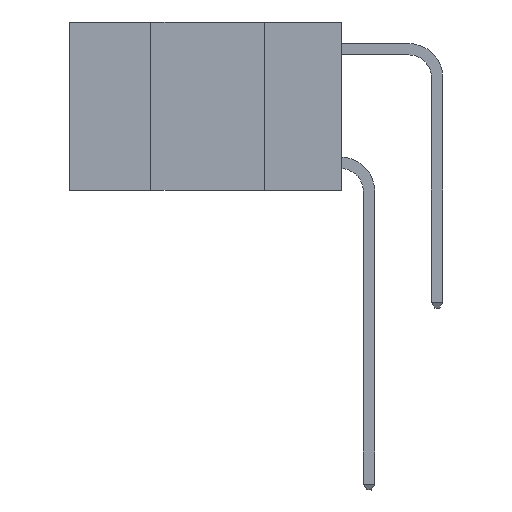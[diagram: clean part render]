
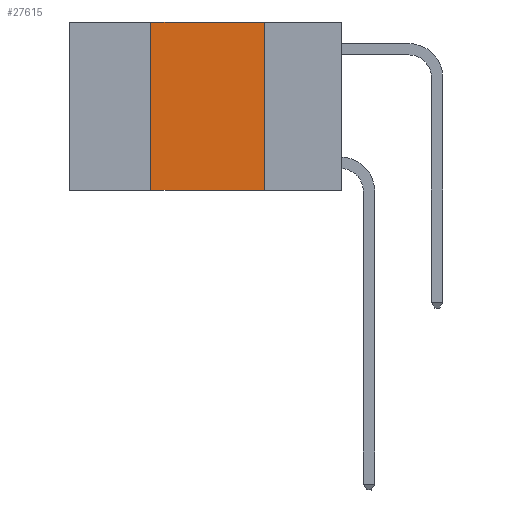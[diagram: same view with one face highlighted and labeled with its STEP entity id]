
A CAD part, left-side view. The second image highlights one B-rep face of the part: STEP entity #27615.
In plain terms, the highlighted planar face has unit normal (-1, 0, 0).
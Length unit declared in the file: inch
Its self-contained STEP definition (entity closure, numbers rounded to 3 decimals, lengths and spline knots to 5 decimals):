
#727 = CARTESIAN_POINT ( 'NONE',  ( 0., 0.6, 0. ) ) ;
#2746 = CARTESIAN_POINT ( 'NONE',  ( 0., 0.17, -0.37 ) ) ;
#2922 = CARTESIAN_POINT ( 'NONE',  ( 0., 0.17, 0. ) ) ;
#3463 = DIRECTION ( 'NONE',  ( 0., 0., -1. ) ) ;
#4274 = DIRECTION ( 'NONE',  ( 0., 0., -1. ) ) ;
#4362 = EDGE_CURVE ( 'NONE', #26511, #19978, #22070, .T. ) ;
#5049 = CARTESIAN_POINT ( 'NONE',  ( 0., 0.6, -0.37 ) ) ;
#6736 = LINE ( 'NONE', #5049, #15609 ) ;
#6961 = CARTESIAN_POINT ( 'NONE',  ( 0., 0.42, -0.37 ) ) ;
#8359 = VECTOR ( 'NONE', #17853, 39.37008 ) ;
#8516 = EDGE_CURVE ( 'NONE', #19978, #18328, #14137, .T. ) ;
#8931 = ORIENTED_EDGE ( 'NONE', *, *, #4362, .F. ) ;
#9910 = EDGE_LOOP ( 'NONE', ( #20988, #8931, #26822, #24869 ) ) ;
#10308 = CARTESIAN_POINT ( 'NONE',  ( 0., 0.6, 0. ) ) ;
#10584 = PLANE ( 'NONE',  #18427 ) ;
#12519 = LINE ( 'NONE', #15058, #15590 ) ;
#12692 = FACE_OUTER_BOUND ( 'NONE', #9910, .T. ) ;
#13722 = EDGE_CURVE ( 'NONE', #15958, #26511, #12519, .T. ) ;
#14137 = LINE ( 'NONE', #2922, #17377 ) ;
#14573 = CARTESIAN_POINT ( 'NONE',  ( 0., 0.17, 0. ) ) ;
#15058 = CARTESIAN_POINT ( 'NONE',  ( 0., 0.42, 0. ) ) ;
#15590 = VECTOR ( 'NONE', #21094, 39.37008 ) ;
#15609 = VECTOR ( 'NONE', #19797, 39.37008 ) ;
#15690 = EDGE_CURVE ( 'NONE', #15958, #18328, #6736, .T. ) ;
#15958 = VERTEX_POINT ( 'NONE', #6961 ) ;
#17377 = VECTOR ( 'NONE', #3463, 39.37008 ) ;
#17853 = DIRECTION ( 'NONE',  ( 0., -1., 0. ) ) ;
#18328 = VERTEX_POINT ( 'NONE', #2746 ) ;
#18427 = AXIS2_PLACEMENT_3D ( 'NONE', #10308, #19292, #4274 ) ;
#19292 = DIRECTION ( 'NONE',  ( 1., 0., 0. ) ) ;
#19797 = DIRECTION ( 'NONE',  ( 0., -1., 0. ) ) ;
#19978 = VERTEX_POINT ( 'NONE', #14573 ) ;
#20988 = ORIENTED_EDGE ( 'NONE', *, *, #8516, .F. ) ;
#21094 = DIRECTION ( 'NONE',  ( 0., 0., 1. ) ) ;
#22070 = LINE ( 'NONE', #727, #8359 ) ;
#22505 = CARTESIAN_POINT ( 'NONE',  ( 0., 0.42, 0. ) ) ;
#24869 = ORIENTED_EDGE ( 'NONE', *, *, #15690, .T. ) ;
#26511 = VERTEX_POINT ( 'NONE', #22505 ) ;
#26822 = ORIENTED_EDGE ( 'NONE', *, *, #13722, .F. ) ;
#27615 = ADVANCED_FACE ( 'NONE', ( #12692 ), #10584, .F. ) ;
